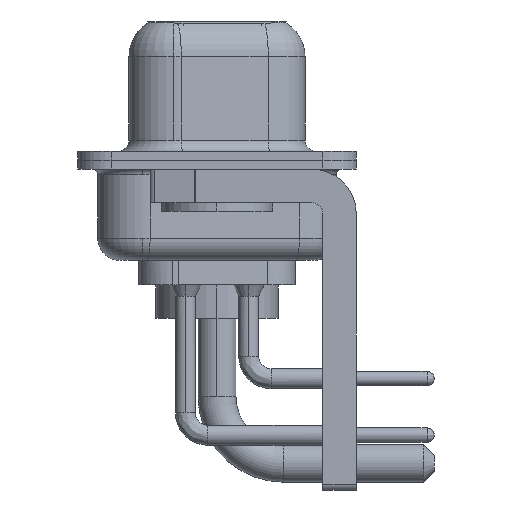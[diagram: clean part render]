
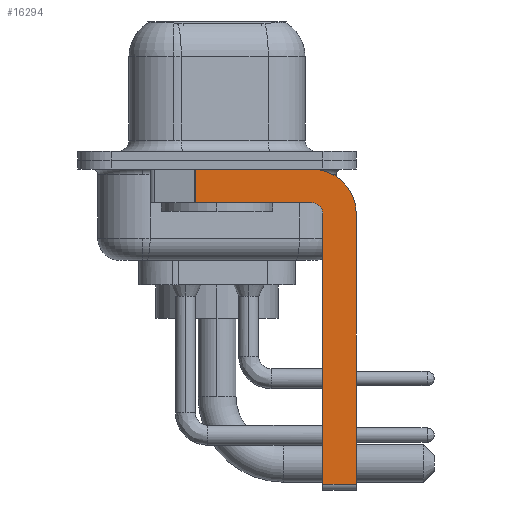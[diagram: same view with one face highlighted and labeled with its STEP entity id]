
A CAD part, left-side view. The second image highlights one B-rep face of the part: STEP entity #16294.
In plain terms, the highlighted planar face has unit normal (-1, 0, 0).
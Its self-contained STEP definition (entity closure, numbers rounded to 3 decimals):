
#210 = ORIENTED_EDGE ( 'NONE', *, *, #14876, .F. ) ;
#643 = VERTEX_POINT ( 'NONE', #4705 ) ;
#1138 = CARTESIAN_POINT ( 'NONE',  ( -2.9, 0.978, -1.9 ) ) ;
#1316 = LINE ( 'NONE', #5285, #15114 ) ;
#1457 = CARTESIAN_POINT ( 'NONE',  ( -2.9, 3., -0.4 ) ) ;
#1490 = EDGE_CURVE ( 'NONE', #14020, #2539, #7644, .T. ) ;
#1793 = CARTESIAN_POINT ( 'NONE',  ( -2.9, -4.25, -14.55 ) ) ;
#2539 = VERTEX_POINT ( 'NONE', #3129 ) ;
#2850 = DIRECTION ( 'NONE',  ( 0., 0., 1. ) ) ;
#3129 = CARTESIAN_POINT ( 'NONE',  ( -2.9, -4.25, -1.9 ) ) ;
#3756 = DIRECTION ( 'NONE',  ( 1., 0., 0. ) ) ;
#4477 = VERTEX_POINT ( 'NONE', #15258 ) ;
#4669 = CARTESIAN_POINT ( 'NONE',  ( -2.9, -4.25, -2.4 ) ) ;
#4705 = CARTESIAN_POINT ( 'NONE',  ( -2.9, 0.978, -0.4 ) ) ;
#4900 = ORIENTED_EDGE ( 'NONE', *, *, #11308, .F. ) ;
#5010 = EDGE_CURVE ( 'NONE', #643, #8185, #7719, .T. ) ;
#5238 = EDGE_LOOP ( 'NONE', ( #7375, #10923, #4900, #6458, #8494, #14627, #15416, #210 ) ) ;
#5285 = CARTESIAN_POINT ( 'NONE',  ( -2.9, -6.25, -2.4 ) ) ;
#5450 = LINE ( 'NONE', #12026, #13607 ) ;
#5454 = VERTEX_POINT ( 'NONE', #13036 ) ;
#5733 = CIRCLE ( 'NONE', #8496, 2. ) ;
#6458 = ORIENTED_EDGE ( 'NONE', *, *, #1490, .F. ) ;
#6729 = DIRECTION ( 'NONE',  ( 0., -1., 0. ) ) ;
#6956 = CARTESIAN_POINT ( 'NONE',  ( -2.9, 0.978, -1.9 ) ) ;
#7206 = EDGE_CURVE ( 'NONE', #15719, #14020, #5450, .T. ) ;
#7375 = ORIENTED_EDGE ( 'NONE', *, *, #9916, .F. ) ;
#7644 = CIRCLE ( 'NONE', #12609, 0.5 ) ;
#7719 = LINE ( 'NONE', #1138, #10455 ) ;
#8185 = VERTEX_POINT ( 'NONE', #6956 ) ;
#8361 = VERTEX_POINT ( 'NONE', #16580 ) ;
#8408 = VECTOR ( 'NONE', #6729, 1000. ) ;
#8494 = ORIENTED_EDGE ( 'NONE', *, *, #7206, .F. ) ;
#8496 = AXIS2_PLACEMENT_3D ( 'NONE', #10335, #3756, #9043 ) ;
#9043 = DIRECTION ( 'NONE',  ( 0., 0., -1. ) ) ;
#9045 = FACE_OUTER_BOUND ( 'NONE', #5238, .T. ) ;
#9502 = LINE ( 'NONE', #11150, #13382 ) ;
#9775 = DIRECTION ( 'NONE',  ( 1., 0., 0. ) ) ;
#9916 = EDGE_CURVE ( 'NONE', #643, #4477, #13292, .T. ) ;
#10335 = CARTESIAN_POINT ( 'NONE',  ( -2.9, -4.25, -2.4 ) ) ;
#10455 = VECTOR ( 'NONE', #15564, 1000. ) ;
#10923 = ORIENTED_EDGE ( 'NONE', *, *, #5010, .T. ) ;
#10953 = DIRECTION ( 'NONE',  ( 0., -1., 0. ) ) ;
#10983 = DIRECTION ( 'NONE',  ( -1., 0., 0. ) ) ;
#11063 = DIRECTION ( 'NONE',  ( 0., 1., 0. ) ) ;
#11150 = CARTESIAN_POINT ( 'NONE',  ( -2.9, -4.25, -1.9 ) ) ;
#11222 = VECTOR ( 'NONE', #10953, 1000. ) ;
#11261 = CARTESIAN_POINT ( 'NONE',  ( -2.9, -4.75, -14.55 ) ) ;
#11308 = EDGE_CURVE ( 'NONE', #2539, #8185, #9502, .T. ) ;
#11518 = DIRECTION ( 'NONE',  ( 0., 0., -1. ) ) ;
#11634 = DIRECTION ( 'NONE',  ( 0., 0., -1. ) ) ;
#11864 = EDGE_CURVE ( 'NONE', #15719, #5454, #12169, .T. ) ;
#12026 = CARTESIAN_POINT ( 'NONE',  ( -2.9, -4.75, -14.8 ) ) ;
#12169 = LINE ( 'NONE', #1793, #11222 ) ;
#12523 = EDGE_CURVE ( 'NONE', #8361, #5454, #1316, .T. ) ;
#12547 = DIRECTION ( 'NONE',  ( 0., 0., 1. ) ) ;
#12609 = AXIS2_PLACEMENT_3D ( 'NONE', #4669, #10983, #12547 ) ;
#13036 = CARTESIAN_POINT ( 'NONE',  ( -2.9, -6.25, -14.55 ) ) ;
#13292 = LINE ( 'NONE', #1457, #8408 ) ;
#13382 = VECTOR ( 'NONE', #11063, 1000. ) ;
#13607 = VECTOR ( 'NONE', #2850, 1000. ) ;
#13753 = PLANE ( 'NONE',  #15425 ) ;
#14020 = VERTEX_POINT ( 'NONE', #16454 ) ;
#14627 = ORIENTED_EDGE ( 'NONE', *, *, #11864, .T. ) ;
#14876 = EDGE_CURVE ( 'NONE', #4477, #8361, #5733, .T. ) ;
#15050 = CARTESIAN_POINT ( 'NONE',  ( -2.9, -4.25, -2.4 ) ) ;
#15114 = VECTOR ( 'NONE', #11518, 1000. ) ;
#15258 = CARTESIAN_POINT ( 'NONE',  ( -2.9, -4.25, -0.4 ) ) ;
#15416 = ORIENTED_EDGE ( 'NONE', *, *, #12523, .F. ) ;
#15425 = AXIS2_PLACEMENT_3D ( 'NONE', #15050, #9775, #11634 ) ;
#15564 = DIRECTION ( 'NONE',  ( 0., 0., -1. ) ) ;
#15719 = VERTEX_POINT ( 'NONE', #11261 ) ;
#16294 = ADVANCED_FACE ( 'NONE', ( #9045 ), #13753, .F. ) ;
#16454 = CARTESIAN_POINT ( 'NONE',  ( -2.9, -4.75, -2.4 ) ) ;
#16580 = CARTESIAN_POINT ( 'NONE',  ( -2.9, -6.25, -2.4 ) ) ;
